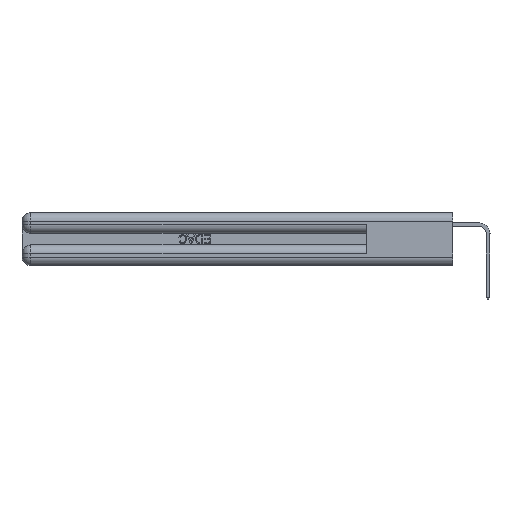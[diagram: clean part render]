
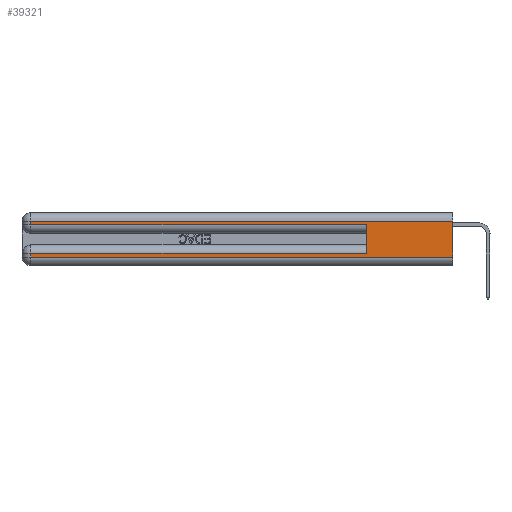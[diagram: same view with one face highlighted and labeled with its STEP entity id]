
A CAD part, left-side view. The second image highlights one B-rep face of the part: STEP entity #39321.
In plain terms, the highlighted planar face has unit normal (-1, 0, 0).
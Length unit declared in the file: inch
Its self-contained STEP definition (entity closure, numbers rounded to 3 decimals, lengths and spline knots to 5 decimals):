
#463 = VERTEX_POINT ( 'NONE', #21787 ) ;
#526 = EDGE_LOOP ( 'NONE', ( #20866, #6293, #24461, #10231, #1460, #24188, #31609, #23904 ) ) ;
#1460 = ORIENTED_EDGE ( 'NONE', *, *, #35340, .F. ) ;
#1638 = LINE ( 'NONE', #28628, #34705 ) ;
#2675 = VERTEX_POINT ( 'NONE', #10593 ) ;
#4364 = VECTOR ( 'NONE', #7149, 39.37008 ) ;
#6089 = EDGE_CURVE ( 'NONE', #39579, #25082, #20065, .T. ) ;
#6162 = DIRECTION ( 'NONE',  ( 0., 0., -1. ) ) ;
#6175 = DIRECTION ( 'NONE',  ( 0., -1., 0. ) ) ;
#6293 = ORIENTED_EDGE ( 'NONE', *, *, #38593, .T. ) ;
#6341 = LINE ( 'NONE', #40167, #21403 ) ;
#6638 = VERTEX_POINT ( 'NONE', #12586 ) ;
#6913 = CARTESIAN_POINT ( 'NONE',  ( 0., 0., 0.31 ) ) ;
#7149 = DIRECTION ( 'NONE',  ( 0., -1., 0. ) ) ;
#9348 = CARTESIAN_POINT ( 'NONE',  ( 0., 2.94, 0.37 ) ) ;
#10231 = ORIENTED_EDGE ( 'NONE', *, *, #23065, .T. ) ;
#10593 = CARTESIAN_POINT ( 'NONE',  ( 0., 0., 0.06 ) ) ;
#10656 = DIRECTION ( 'NONE',  ( 1., 0., 0. ) ) ;
#11560 = VECTOR ( 'NONE', #34490, 39.37008 ) ;
#12017 = VERTEX_POINT ( 'NONE', #36251 ) ;
#12586 = CARTESIAN_POINT ( 'NONE',  ( 0., 2.94, 0.31 ) ) ;
#13055 = VERTEX_POINT ( 'NONE', #31625 ) ;
#13918 = LINE ( 'NONE', #20053, #4364 ) ;
#14298 = LINE ( 'NONE', #37944, #36800 ) ;
#18214 = VERTEX_POINT ( 'NONE', #26317 ) ;
#18567 = CARTESIAN_POINT ( 'NONE',  ( 0., 0., 0.085 ) ) ;
#18881 = VECTOR ( 'NONE', #32558, 39.37008 ) ;
#19237 = EDGE_CURVE ( 'NONE', #18214, #2675, #1638, .T. ) ;
#20047 = DIRECTION ( 'NONE',  ( 0., 0., -1. ) ) ;
#20053 = CARTESIAN_POINT ( 'NONE',  ( 0., 0., 0.285 ) ) ;
#20065 = LINE ( 'NONE', #18567, #11560 ) ;
#20866 = ORIENTED_EDGE ( 'NONE', *, *, #24705, .F. ) ;
#20915 = VECTOR ( 'NONE', #20047, 39.37008 ) ;
#21403 = VECTOR ( 'NONE', #33882, 39.37008 ) ;
#21787 = CARTESIAN_POINT ( 'NONE',  ( 0., 0.6, 0.285 ) ) ;
#23065 = EDGE_CURVE ( 'NONE', #12017, #463, #13918, .T. ) ;
#23904 = ORIENTED_EDGE ( 'NONE', *, *, #19237, .T. ) ;
#24188 = ORIENTED_EDGE ( 'NONE', *, *, #6089, .T. ) ;
#24461 = ORIENTED_EDGE ( 'NONE', *, *, #35102, .T. ) ;
#24705 = EDGE_CURVE ( 'NONE', #13055, #2675, #14298, .T. ) ;
#24784 = CARTESIAN_POINT ( 'NONE',  ( 0., 2.94, 0.085 ) ) ;
#25082 = VERTEX_POINT ( 'NONE', #24784 ) ;
#25460 = DIRECTION ( 'NONE',  ( 0., 0., -1. ) ) ;
#26317 = CARTESIAN_POINT ( 'NONE',  ( 0., 2.94, 0.06 ) ) ;
#26384 = LINE ( 'NONE', #6913, #18881 ) ;
#27014 = EDGE_CURVE ( 'NONE', #25082, #18214, #40150, .T. ) ;
#28004 = CARTESIAN_POINT ( 'NONE',  ( 0., 0.6, 0.085 ) ) ;
#28628 = CARTESIAN_POINT ( 'NONE',  ( 0., 0., 0.06 ) ) ;
#29448 = LINE ( 'NONE', #32776, #20915 ) ;
#29844 = CARTESIAN_POINT ( 'NONE',  ( 0., 0., 0.37 ) ) ;
#31609 = ORIENTED_EDGE ( 'NONE', *, *, #27014, .T. ) ;
#31625 = CARTESIAN_POINT ( 'NONE',  ( 0., 0., 0.31 ) ) ;
#32558 = DIRECTION ( 'NONE',  ( 0., 1., 0. ) ) ;
#32776 = CARTESIAN_POINT ( 'NONE',  ( 0., 2.94, 0.37 ) ) ;
#33027 = DIRECTION ( 'NONE',  ( 0., 0., -1. ) ) ;
#33882 = DIRECTION ( 'NONE',  ( 0., 0., 1. ) ) ;
#34073 = AXIS2_PLACEMENT_3D ( 'NONE', #29844, #10656, #33027 ) ;
#34490 = DIRECTION ( 'NONE',  ( 0., 1., 0. ) ) ;
#34705 = VECTOR ( 'NONE', #6175, 39.37008 ) ;
#35102 = EDGE_CURVE ( 'NONE', #6638, #12017, #29448, .T. ) ;
#35340 = EDGE_CURVE ( 'NONE', #39579, #463, #6341, .T. ) ;
#36251 = CARTESIAN_POINT ( 'NONE',  ( 0., 2.94, 0.285 ) ) ;
#36800 = VECTOR ( 'NONE', #6162, 39.37008 ) ;
#37944 = CARTESIAN_POINT ( 'NONE',  ( 0., 0., 0.37 ) ) ;
#38593 = EDGE_CURVE ( 'NONE', #13055, #6638, #26384, .T. ) ;
#39321 = ADVANCED_FACE ( 'NONE', ( #40825 ), #39324, .F. ) ;
#39324 = PLANE ( 'NONE',  #34073 ) ;
#39579 = VERTEX_POINT ( 'NONE', #28004 ) ;
#40150 = LINE ( 'NONE', #9348, #41151 ) ;
#40167 = CARTESIAN_POINT ( 'NONE',  ( 0., 0.6, 0.145 ) ) ;
#40825 = FACE_OUTER_BOUND ( 'NONE', #526, .T. ) ;
#41151 = VECTOR ( 'NONE', #25460, 39.37008 ) ;
